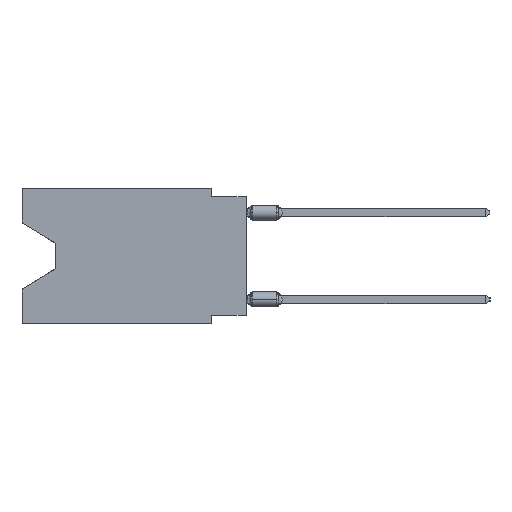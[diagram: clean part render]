
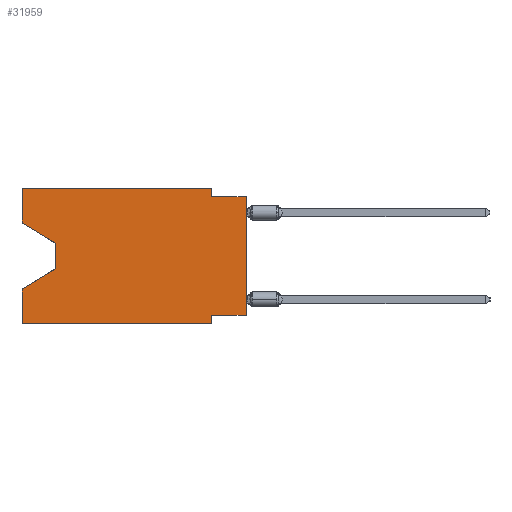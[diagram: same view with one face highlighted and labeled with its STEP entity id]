
A CAD part, left-side view. The second image highlights one B-rep face of the part: STEP entity #31959.
In plain terms, the highlighted planar face has unit normal (-1, 0, 0).
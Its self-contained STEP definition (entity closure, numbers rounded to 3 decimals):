
#228 = VECTOR ( 'NONE', #14688, 1000. ) ;
#325 = VECTOR ( 'NONE', #20022, 1000. ) ;
#734 = VERTEX_POINT ( 'NONE', #24969 ) ;
#1902 = DIRECTION ( 'NONE',  ( 0., 1., 0. ) ) ;
#1931 = VECTOR ( 'NONE', #9979, 1000. ) ;
#2294 = ORIENTED_EDGE ( 'NONE', *, *, #24569, .T. ) ;
#2472 = VERTEX_POINT ( 'NONE', #34384 ) ;
#2791 = LINE ( 'NONE', #32899, #19194 ) ;
#3329 = CARTESIAN_POINT ( 'NONE',  ( 0., 2.54, 0. ) ) ;
#3655 = EDGE_CURVE ( 'NONE', #33550, #7240, #20537, .T. ) ;
#3766 = LINE ( 'NONE', #25971, #228 ) ;
#3788 = EDGE_CURVE ( 'NONE', #2472, #27901, #2791, .T. ) ;
#4058 = DIRECTION ( 'NONE',  ( 0., 0., 1. ) ) ;
#4596 = VERTEX_POINT ( 'NONE', #32811 ) ;
#5533 = CARTESIAN_POINT ( 'NONE',  ( 0., 13.97, -5.893 ) ) ;
#5649 = LINE ( 'NONE', #9353, #31903 ) ;
#5798 = ORIENTED_EDGE ( 'NONE', *, *, #21575, .T. ) ;
#5816 = DIRECTION ( 'NONE',  ( 0., -0.855, -0.519 ) ) ;
#6054 = VECTOR ( 'NONE', #1902, 1000. ) ;
#6137 = EDGE_CURVE ( 'NONE', #7240, #734, #5649, .T. ) ;
#6287 = DIRECTION ( 'NONE',  ( 1., 0., 0. ) ) ;
#6366 = LINE ( 'NONE', #28044, #24250 ) ;
#6772 = CARTESIAN_POINT ( 'NONE',  ( 0., 2.54, -9.271 ) ) ;
#6929 = CARTESIAN_POINT ( 'NONE',  ( 0., 0., -9.271 ) ) ;
#7144 = CARTESIAN_POINT ( 'NONE',  ( 0., 13.97, -4.013 ) ) ;
#7206 = VERTEX_POINT ( 'NONE', #23058 ) ;
#7240 = VERTEX_POINT ( 'NONE', #6772 ) ;
#8657 = VERTEX_POINT ( 'NONE', #8705 ) ;
#8705 = CARTESIAN_POINT ( 'NONE',  ( 0., 16.383, 0. ) ) ;
#8738 = EDGE_CURVE ( 'NONE', #8657, #17049, #6366, .T. ) ;
#8969 = DIRECTION ( 'NONE',  ( 0., 0., 1. ) ) ;
#9208 = ORIENTED_EDGE ( 'NONE', *, *, #3655, .F. ) ;
#9353 = CARTESIAN_POINT ( 'NONE',  ( 0., 2.54, -9.906 ) ) ;
#9628 = CARTESIAN_POINT ( 'NONE',  ( 0., 0., 0. ) ) ;
#9979 = DIRECTION ( 'NONE',  ( 0., -1., 0. ) ) ;
#10667 = ORIENTED_EDGE ( 'NONE', *, *, #17681, .T. ) ;
#11112 = ORIENTED_EDGE ( 'NONE', *, *, #3788, .T. ) ;
#11389 = LINE ( 'NONE', #3329, #35096 ) ;
#12018 = EDGE_CURVE ( 'NONE', #23873, #33233, #20631, .T. ) ;
#12571 = DIRECTION ( 'NONE',  ( 0., -1., 0. ) ) ;
#12625 = EDGE_CURVE ( 'NONE', #2472, #8657, #22557, .T. ) ;
#12990 = ORIENTED_EDGE ( 'NONE', *, *, #31038, .F. ) ;
#13581 = CARTESIAN_POINT ( 'NONE',  ( 0., 0., -0.635 ) ) ;
#14090 = VECTOR ( 'NONE', #12571, 1000. ) ;
#14688 = DIRECTION ( 'NONE',  ( 0., 0., -1. ) ) ;
#15848 = VERTEX_POINT ( 'NONE', #20548 ) ;
#17049 = VERTEX_POINT ( 'NONE', #19358 ) ;
#17073 = ORIENTED_EDGE ( 'NONE', *, *, #12018, .F. ) ;
#17681 = EDGE_CURVE ( 'NONE', #15848, #734, #31142, .T. ) ;
#17682 = LINE ( 'NONE', #9628, #34496 ) ;
#19139 = LINE ( 'NONE', #5533, #20351 ) ;
#19179 = CARTESIAN_POINT ( 'NONE',  ( 0., 16.383, 0. ) ) ;
#19194 = VECTOR ( 'NONE', #5816, 1000. ) ;
#19196 = EDGE_CURVE ( 'NONE', #27901, #4596, #3766, .T. ) ;
#19348 = LINE ( 'NONE', #19179, #30093 ) ;
#19358 = CARTESIAN_POINT ( 'NONE',  ( 0., 2.54, 0. ) ) ;
#19890 = CARTESIAN_POINT ( 'NONE',  ( 0., 16.383, 0. ) ) ;
#20022 = DIRECTION ( 'NONE',  ( 0., 0., 1. ) ) ;
#20351 = VECTOR ( 'NONE', #30083, 1000. ) ;
#20537 = LINE ( 'NONE', #6929, #6054 ) ;
#20548 = CARTESIAN_POINT ( 'NONE',  ( 0., 16.383, -9.906 ) ) ;
#20631 = LINE ( 'NONE', #29430, #14090 ) ;
#21466 = ORIENTED_EDGE ( 'NONE', *, *, #12625, .F. ) ;
#21575 = EDGE_CURVE ( 'NONE', #33550, #33233, #17682, .T. ) ;
#22557 = LINE ( 'NONE', #32975, #325 ) ;
#22674 = DIRECTION ( 'NONE',  ( 0., -1., 0. ) ) ;
#22690 = ORIENTED_EDGE ( 'NONE', *, *, #6137, .F. ) ;
#22759 = FACE_OUTER_BOUND ( 'NONE', #28302, .T. ) ;
#23058 = CARTESIAN_POINT ( 'NONE',  ( 0., 16.383, -7.36 ) ) ;
#23873 = VERTEX_POINT ( 'NONE', #34251 ) ;
#24118 = EDGE_CURVE ( 'NONE', #15848, #7206, #19348, .T. ) ;
#24250 = VECTOR ( 'NONE', #22674, 1000. ) ;
#24488 = DIRECTION ( 'NONE',  ( 0., 0., -1. ) ) ;
#24569 = EDGE_CURVE ( 'NONE', #4596, #7206, #19139, .T. ) ;
#24969 = CARTESIAN_POINT ( 'NONE',  ( 0., 2.54, -9.906 ) ) ;
#25336 = ORIENTED_EDGE ( 'NONE', *, *, #19196, .T. ) ;
#25971 = CARTESIAN_POINT ( 'NONE',  ( 0., 13.97, -4.013 ) ) ;
#27901 = VERTEX_POINT ( 'NONE', #7144 ) ;
#28044 = CARTESIAN_POINT ( 'NONE',  ( 0., 16.383, 0. ) ) ;
#28302 = EDGE_LOOP ( 'NONE', ( #11112, #25336, #2294, #30368, #10667, #22690, #9208, #5798, #17073, #12990, #29621, #21466 ) ) ;
#28513 = DIRECTION ( 'NONE',  ( 0., 0., -1. ) ) ;
#29430 = CARTESIAN_POINT ( 'NONE',  ( 0., 0., -0.635 ) ) ;
#29621 = ORIENTED_EDGE ( 'NONE', *, *, #8738, .F. ) ;
#30083 = DIRECTION ( 'NONE',  ( 0., 0.855, -0.519 ) ) ;
#30093 = VECTOR ( 'NONE', #8969, 1000. ) ;
#30368 = ORIENTED_EDGE ( 'NONE', *, *, #24118, .F. ) ;
#30410 = CARTESIAN_POINT ( 'NONE',  ( 0., 0., -9.271 ) ) ;
#31038 = EDGE_CURVE ( 'NONE', #17049, #23873, #11389, .T. ) ;
#31142 = LINE ( 'NONE', #31849, #1931 ) ;
#31849 = CARTESIAN_POINT ( 'NONE',  ( 0., 16.383, -9.906 ) ) ;
#31903 = VECTOR ( 'NONE', #28513, 1000. ) ;
#31959 = ADVANCED_FACE ( 'NONE', ( #22759 ), #33529, .F. ) ;
#32811 = CARTESIAN_POINT ( 'NONE',  ( 0., 13.97, -5.893 ) ) ;
#32899 = CARTESIAN_POINT ( 'NONE',  ( 0., 16.383, -2.546 ) ) ;
#32975 = CARTESIAN_POINT ( 'NONE',  ( 0., 16.383, 0. ) ) ;
#33233 = VERTEX_POINT ( 'NONE', #13581 ) ;
#33529 = PLANE ( 'NONE',  #34561 ) ;
#33550 = VERTEX_POINT ( 'NONE', #30410 ) ;
#33695 = DIRECTION ( 'NONE',  ( 0., 0., -1. ) ) ;
#34251 = CARTESIAN_POINT ( 'NONE',  ( 0., 2.54, -0.635 ) ) ;
#34384 = CARTESIAN_POINT ( 'NONE',  ( 0., 16.383, -2.546 ) ) ;
#34496 = VECTOR ( 'NONE', #4058, 1000. ) ;
#34561 = AXIS2_PLACEMENT_3D ( 'NONE', #19890, #6287, #33695 ) ;
#35096 = VECTOR ( 'NONE', #24488, 1000. ) ;
